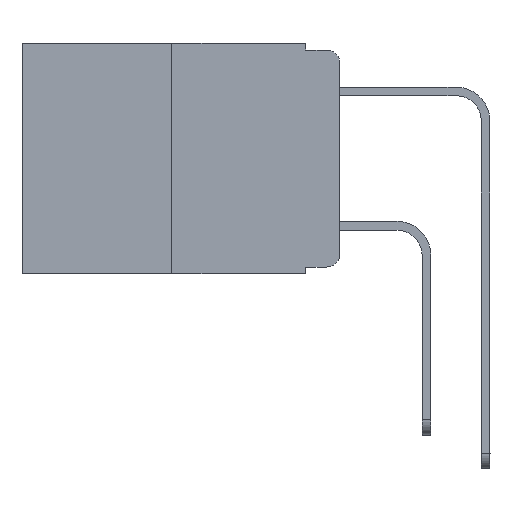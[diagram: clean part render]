
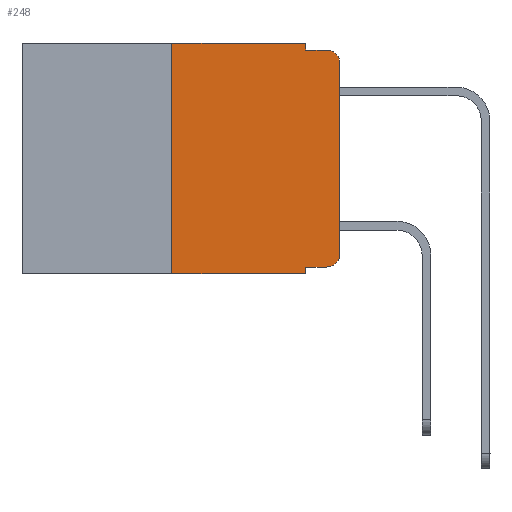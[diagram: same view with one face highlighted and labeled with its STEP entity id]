
A CAD part, left-side view. The second image highlights one B-rep face of the part: STEP entity #248.
In plain terms, the highlighted planar face has unit normal (-1, 0, 0).
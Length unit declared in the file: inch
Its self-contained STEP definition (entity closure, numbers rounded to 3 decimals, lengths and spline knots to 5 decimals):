
#38 = LINE ( 'NONE', #14505, #14274 ) ;
#49 = EDGE_CURVE ( 'NONE', #13851, #10990, #16449, .T. ) ;
#248 = ADVANCED_FACE ( 'NONE', ( #8437 ), #14973, .F. ) ;
#1136 = ORIENTED_EDGE ( 'NONE', *, *, #6936, .F. ) ;
#1581 = CARTESIAN_POINT ( 'NONE',  ( 0., 0.473, 0. ) ) ;
#1724 = CARTESIAN_POINT ( 'NONE',  ( 0., 0.25, 0. ) ) ;
#1784 = EDGE_LOOP ( 'NONE', ( #8612, #2582, #2280, #14208, #8632, #16238, #9099, #1136, #12713, #10056 ) ) ;
#1785 = VECTOR ( 'NONE', #7817, 39.37008 ) ;
#1874 = CARTESIAN_POINT ( 'NONE',  ( 0., 0.473, 0. ) ) ;
#1949 = VERTEX_POINT ( 'NONE', #5195 ) ;
#2280 = ORIENTED_EDGE ( 'NONE', *, *, #9152, .F. ) ;
#2522 = LINE ( 'NONE', #6309, #15799 ) ;
#2582 = ORIENTED_EDGE ( 'NONE', *, *, #49, .T. ) ;
#3355 = DIRECTION ( 'NONE',  ( 1., 0., 0. ) ) ;
#3411 = LINE ( 'NONE', #12709, #15439 ) ;
#3464 = CIRCLE ( 'NONE', #9230, 0.02 ) ;
#3625 = DIRECTION ( 'NONE',  ( -1., 0., 0. ) ) ;
#4002 = VECTOR ( 'NONE', #5493, 39.37008 ) ;
#4183 = VECTOR ( 'NONE', #13216, 39.37008 ) ;
#4202 = CARTESIAN_POINT ( 'NONE',  ( 0., 0.02, -0.333 ) ) ;
#4962 = CARTESIAN_POINT ( 'NONE',  ( 0., 0.051, 0. ) ) ;
#5020 = EDGE_CURVE ( 'NONE', #12861, #16097, #14197, .T. ) ;
#5195 = CARTESIAN_POINT ( 'NONE',  ( 0., 0., -0.313 ) ) ;
#5493 = DIRECTION ( 'NONE',  ( 0., 0., 1. ) ) ;
#5582 = VERTEX_POINT ( 'NONE', #7964 ) ;
#5967 = CARTESIAN_POINT ( 'NONE',  ( 0., 0.25, -0.343 ) ) ;
#6309 = CARTESIAN_POINT ( 'NONE',  ( 0., 0.473, -0.343 ) ) ;
#6632 = VECTOR ( 'NONE', #12120, 39.37008 ) ;
#6936 = EDGE_CURVE ( 'NONE', #15336, #5582, #10552, .T. ) ;
#7233 = LINE ( 'NONE', #14893, #4002 ) ;
#7817 = DIRECTION ( 'NONE',  ( 0., 0., -1. ) ) ;
#7906 = EDGE_CURVE ( 'NONE', #1949, #13851, #7233, .T. ) ;
#7964 = CARTESIAN_POINT ( 'NONE',  ( 0., 0.051, -0.343 ) ) ;
#8357 = CARTESIAN_POINT ( 'NONE',  ( 0., 0.051, 0. ) ) ;
#8437 = FACE_OUTER_BOUND ( 'NONE', #1784, .T. ) ;
#8612 = ORIENTED_EDGE ( 'NONE', *, *, #7906, .T. ) ;
#8632 = ORIENTED_EDGE ( 'NONE', *, *, #11701, .F. ) ;
#8659 = DIRECTION ( 'NONE',  ( 0., -1., 0. ) ) ;
#9072 = VERTEX_POINT ( 'NONE', #1724 ) ;
#9099 = ORIENTED_EDGE ( 'NONE', *, *, #15373, .T. ) ;
#9152 = EDGE_CURVE ( 'NONE', #16097, #10990, #38, .T. ) ;
#9230 = AXIS2_PLACEMENT_3D ( 'NONE', #11792, #14440, #11714 ) ;
#9644 = DIRECTION ( 'NONE',  ( 0., 0., -1. ) ) ;
#9678 = CARTESIAN_POINT ( 'NONE',  ( 0., 0.02, -0.01 ) ) ;
#9853 = EDGE_CURVE ( 'NONE', #14145, #1949, #3464, .T. ) ;
#10056 = ORIENTED_EDGE ( 'NONE', *, *, #9853, .T. ) ;
#10163 = AXIS2_PLACEMENT_3D ( 'NONE', #1874, #3355, #9644 ) ;
#10552 = LINE ( 'NONE', #13472, #12394 ) ;
#10555 = DIRECTION ( 'NONE',  ( 0., -1., 0. ) ) ;
#10731 = LINE ( 'NONE', #1581, #6632 ) ;
#10990 = VERTEX_POINT ( 'NONE', #9678 ) ;
#11566 = DIRECTION ( 'NONE',  ( 0., -1., 0. ) ) ;
#11701 = EDGE_CURVE ( 'NONE', #9072, #12861, #10731, .T. ) ;
#11714 = DIRECTION ( 'NONE',  ( 0., 0., -1. ) ) ;
#11792 = CARTESIAN_POINT ( 'NONE',  ( 0., 0.02, -0.313 ) ) ;
#11960 = EDGE_CURVE ( 'NONE', #15336, #14145, #3411, .T. ) ;
#12120 = DIRECTION ( 'NONE',  ( 0., -1., 0. ) ) ;
#12197 = CARTESIAN_POINT ( 'NONE',  ( 0., 0.25, 0. ) ) ;
#12394 = VECTOR ( 'NONE', #14586, 39.37008 ) ;
#12684 = CARTESIAN_POINT ( 'NONE',  ( 0., 0.051, -0.333 ) ) ;
#12709 = CARTESIAN_POINT ( 'NONE',  ( 0., 0.051, -0.333 ) ) ;
#12713 = ORIENTED_EDGE ( 'NONE', *, *, #11960, .T. ) ;
#12861 = VERTEX_POINT ( 'NONE', #8357 ) ;
#13216 = DIRECTION ( 'NONE',  ( 0., 0., 1. ) ) ;
#13400 = EDGE_CURVE ( 'NONE', #15264, #9072, #15873, .T. ) ;
#13425 = DIRECTION ( 'NONE',  ( 0., 0., -1. ) ) ;
#13427 = AXIS2_PLACEMENT_3D ( 'NONE', #15417, #3625, #13425 ) ;
#13472 = CARTESIAN_POINT ( 'NONE',  ( 0., 0.051, 0. ) ) ;
#13851 = VERTEX_POINT ( 'NONE', #15168 ) ;
#13852 = CARTESIAN_POINT ( 'NONE',  ( 0., 0.051, -0.01 ) ) ;
#14145 = VERTEX_POINT ( 'NONE', #4202 ) ;
#14197 = LINE ( 'NONE', #4962, #1785 ) ;
#14208 = ORIENTED_EDGE ( 'NONE', *, *, #5020, .F. ) ;
#14274 = VECTOR ( 'NONE', #10555, 39.37008 ) ;
#14440 = DIRECTION ( 'NONE',  ( -1., 0., 0. ) ) ;
#14505 = CARTESIAN_POINT ( 'NONE',  ( 0., 0.051, -0.01 ) ) ;
#14586 = DIRECTION ( 'NONE',  ( 0., 0., -1. ) ) ;
#14893 = CARTESIAN_POINT ( 'NONE',  ( 0., 0., 0. ) ) ;
#14973 = PLANE ( 'NONE',  #10163 ) ;
#15168 = CARTESIAN_POINT ( 'NONE',  ( 0., 0., -0.03 ) ) ;
#15264 = VERTEX_POINT ( 'NONE', #5967 ) ;
#15336 = VERTEX_POINT ( 'NONE', #12684 ) ;
#15373 = EDGE_CURVE ( 'NONE', #15264, #5582, #2522, .T. ) ;
#15417 = CARTESIAN_POINT ( 'NONE',  ( 0., 0.02, -0.03 ) ) ;
#15439 = VECTOR ( 'NONE', #8659, 39.37008 ) ;
#15799 = VECTOR ( 'NONE', #11566, 39.37008 ) ;
#15873 = LINE ( 'NONE', #12197, #4183 ) ;
#16097 = VERTEX_POINT ( 'NONE', #13852 ) ;
#16238 = ORIENTED_EDGE ( 'NONE', *, *, #13400, .F. ) ;
#16449 = CIRCLE ( 'NONE', #13427, 0.02 ) ;
